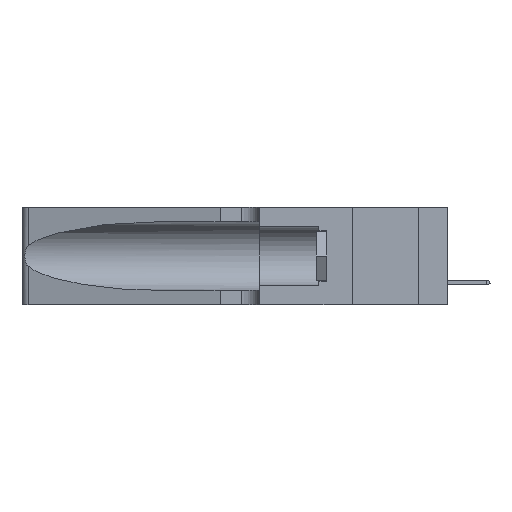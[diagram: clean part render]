
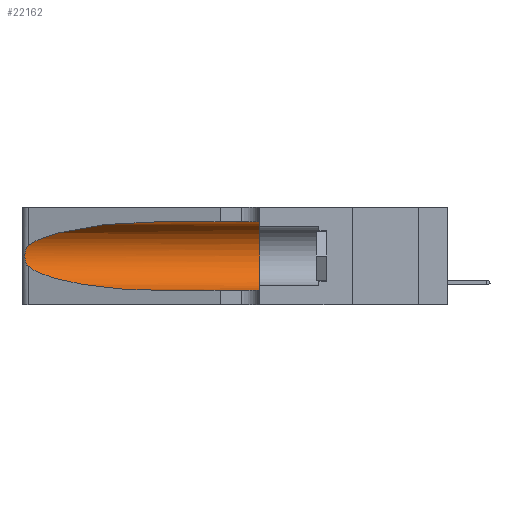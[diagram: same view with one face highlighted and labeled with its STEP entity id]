
A CAD part, left-side view. The second image highlights one B-rep face of the part: STEP entity #22162.
In plain terms, the highlighted cylindrical face has radius 3.308 mm (diameter 6.617 mm), a partial arc.
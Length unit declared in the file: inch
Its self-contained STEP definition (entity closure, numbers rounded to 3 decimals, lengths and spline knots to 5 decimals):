
#684 = CARTESIAN_POINT ( 'NONE',  ( 0.1305, 0.35, 0.05475 ) ) ;
#1386 = CIRCLE ( 'NONE', #19086, 0.13025 ) ;
#1621 = DIRECTION ( 'NONE',  ( 0., 0., -1. ) ) ;
#1824 = EDGE_CURVE ( 'NONE', #25928, #15296, #16652, .T. ) ;
#2349 = CARTESIAN_POINT ( 'NONE',  ( 0.25555, 1.22994, 0.2215 ) ) ;
#3084 = CARTESIAN_POINT ( 'NONE',  ( 0.1305, 0.72297, 0.05475 ) ) ;
#3123 = VERTEX_POINT ( 'NONE', #684 ) ;
#3308 = LINE ( 'NONE', #10110, #9638 ) ;
#3733 = CARTESIAN_POINT ( 'NONE',  ( 0.1305, 0.72297, 0.05475 ) ) ;
#4033 = CARTESIAN_POINT ( 'NONE',  ( 0.18966, 0.96281, 0.05475 ) ) ;
#4996 = DIRECTION ( 'NONE',  ( 0., -1., 0. ) ) ;
#5914 = EDGE_CURVE ( 'NONE', #20063, #3123, #1386, .T. ) ;
#6029 = DIRECTION ( 'NONE',  ( 0., -1., 0. ) ) ;
#6760 = CARTESIAN_POINT ( 'NONE',  ( 0.26075, 1.23896, 0.178 ) ) ;
#6879 = CARTESIAN_POINT ( 'NONE',  ( 0.25487, 1.22718, 0.22369 ) ) ;
#7204 =( BOUNDED_CURVE ( )  B_SPLINE_CURVE ( 3, ( #25616, #7898, #23556, #14413 ),
 .UNSPECIFIED., .F., .F. ) 
 B_SPLINE_CURVE_WITH_KNOTS ( ( 4, 4 ),
 ( 1.5708, 2.84003 ),
 .UNSPECIFIED. ) 
 CURVE ( )  GEOMETRIC_REPRESENTATION_ITEM ( )  RATIONAL_B_SPLINE_CURVE ( ( 1., 0.87, 0.87, 1. ) ) 
 REPRESENTATION_ITEM ( '' )  );
#7898 = CARTESIAN_POINT ( 'NONE',  ( 0.18966, 0.96281, 0.31525 ) ) ;
#8637 = CYLINDRICAL_SURFACE ( 'NONE', #27213, 0.13025 ) ;
#9026 = CARTESIAN_POINT ( 'NONE',  ( 0.25789, 1.23486, 0.15765 ) ) ;
#9638 = VECTOR ( 'NONE', #21412, 39.37008 ) ;
#9672 = CARTESIAN_POINT ( 'NONE',  ( 0.1305, 0.72297, 0.31525 ) ) ;
#10110 = CARTESIAN_POINT ( 'NONE',  ( 0.1305, 1.61858, 0.31525 ) ) ;
#11077 = CARTESIAN_POINT ( 'NONE',  ( 0.25487, 1.22718, 0.14631 ) ) ;
#11184 = CARTESIAN_POINT ( 'NONE',  ( 0.25639, 1.23186, 0.15144 ) ) ;
#11567 = DIRECTION ( 'NONE',  ( 0., 1., 0. ) ) ;
#12574 = CARTESIAN_POINT ( 'NONE',  ( 0.1305, 1.61858, 0.185 ) ) ;
#13070 = EDGE_CURVE ( 'NONE', #15296, #3123, #16694, .T. ) ;
#13120 = CARTESIAN_POINT ( 'NONE',  ( 0.25555, 1.22993, 0.14849 ) ) ;
#14079 = VERTEX_POINT ( 'NONE', #9672 ) ;
#14196 = EDGE_LOOP ( 'NONE', ( #21336, #16766, #15102, #15509, #19518, #16164 ) ) ;
#14413 = CARTESIAN_POINT ( 'NONE',  ( 0.25487, 1.22718, 0.22369 ) ) ;
#14664 = CARTESIAN_POINT ( 'NONE',  ( 0.25487, 1.22718, 0.14631 ) ) ;
#14709 = VERTEX_POINT ( 'NONE', #6879 ) ;
#15102 = ORIENTED_EDGE ( 'NONE', *, *, #1824, .T. ) ;
#15160 = CARTESIAN_POINT ( 'NONE',  ( 0.2373, 1.15595, 0.08982 ) ) ;
#15296 = VERTEX_POINT ( 'NONE', #3084 ) ;
#15421 = B_SPLINE_CURVE_WITH_KNOTS ( 'NONE', 3,
 ( #15725, #2349, #29013, #19834, #24292, #17879, #15533, #6760, #17786, #17967, #9026, #11184, #13120, #11077 ),
 .UNSPECIFIED., .F., .F.,
 ( 4, 2, 2, 2, 2, 2, 4 ),
 ( 0., 0.00027, 0.00053, 0.00107, 0.0016, 0.00187, 0.00214 ),
 .UNSPECIFIED. ) ;
#15509 = ORIENTED_EDGE ( 'NONE', *, *, #13070, .T. ) ;
#15533 = CARTESIAN_POINT ( 'NONE',  ( 0.26075, 1.23896, 0.19203 ) ) ;
#15614 = EDGE_CURVE ( 'NONE', #14079, #14709, #7204, .T. ) ;
#15725 = CARTESIAN_POINT ( 'NONE',  ( 0.25487, 1.22718, 0.22369 ) ) ;
#16164 = ORIENTED_EDGE ( 'NONE', *, *, #22769, .F. ) ;
#16652 =( BOUNDED_CURVE ( )  B_SPLINE_CURVE ( 3, ( #17107, #15160, #4033, #3733 ),
 .UNSPECIFIED., .F., .T. ) 
 B_SPLINE_CURVE_WITH_KNOTS ( ( 4, 4 ),
 ( 3.44316, 4.71239 ),
 .UNSPECIFIED. ) 
 CURVE ( )  GEOMETRIC_REPRESENTATION_ITEM ( )  RATIONAL_B_SPLINE_CURVE ( ( 1., 0.87, 0.87, 1. ) ) 
 REPRESENTATION_ITEM ( '' )  );
#16694 = LINE ( 'NONE', #25143, #28689 ) ;
#16766 = ORIENTED_EDGE ( 'NONE', *, *, #18784, .T. ) ;
#17107 = CARTESIAN_POINT ( 'NONE',  ( 0.25487, 1.22718, 0.14631 ) ) ;
#17786 = CARTESIAN_POINT ( 'NONE',  ( 0.26017, 1.23833, 0.17102 ) ) ;
#17879 = CARTESIAN_POINT ( 'NONE',  ( 0.26018, 1.23835, 0.19895 ) ) ;
#17967 = CARTESIAN_POINT ( 'NONE',  ( 0.25856, 1.23593, 0.16098 ) ) ;
#18784 = EDGE_CURVE ( 'NONE', #14709, #25928, #15421, .T. ) ;
#19086 = AXIS2_PLACEMENT_3D ( 'NONE', #26947, #11567, #27239 ) ;
#19518 = ORIENTED_EDGE ( 'NONE', *, *, #5914, .F. ) ;
#19834 = CARTESIAN_POINT ( 'NONE',  ( 0.25787, 1.23484, 0.2124 ) ) ;
#20063 = VERTEX_POINT ( 'NONE', #24512 ) ;
#21336 = ORIENTED_EDGE ( 'NONE', *, *, #15614, .T. ) ;
#21412 = DIRECTION ( 'NONE',  ( 0., -1., 0. ) ) ;
#22162 = ADVANCED_FACE ( 'NONE', ( #27912 ), #8637, .F. ) ;
#22769 = EDGE_CURVE ( 'NONE', #14079, #20063, #3308, .T. ) ;
#23556 = CARTESIAN_POINT ( 'NONE',  ( 0.2373, 1.15595, 0.28018 ) ) ;
#24292 = CARTESIAN_POINT ( 'NONE',  ( 0.25854, 1.2359, 0.20912 ) ) ;
#24512 = CARTESIAN_POINT ( 'NONE',  ( 0.1305, 0.35, 0.31525 ) ) ;
#25143 = CARTESIAN_POINT ( 'NONE',  ( 0.1305, 1.61858, 0.05475 ) ) ;
#25616 = CARTESIAN_POINT ( 'NONE',  ( 0.1305, 0.72297, 0.31525 ) ) ;
#25928 = VERTEX_POINT ( 'NONE', #14664 ) ;
#26947 = CARTESIAN_POINT ( 'NONE',  ( 0.1305, 0.35, 0.185 ) ) ;
#27213 = AXIS2_PLACEMENT_3D ( 'NONE', #12574, #6029, #1621 ) ;
#27239 = DIRECTION ( 'NONE',  ( 0., 0., 1. ) ) ;
#27912 = FACE_OUTER_BOUND ( 'NONE', #14196, .T. ) ;
#28689 = VECTOR ( 'NONE', #4996, 39.37008 ) ;
#29013 = CARTESIAN_POINT ( 'NONE',  ( 0.25639, 1.23184, 0.21858 ) ) ;
